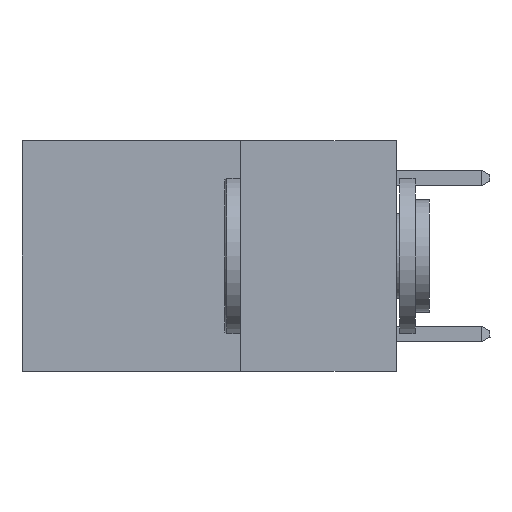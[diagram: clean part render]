
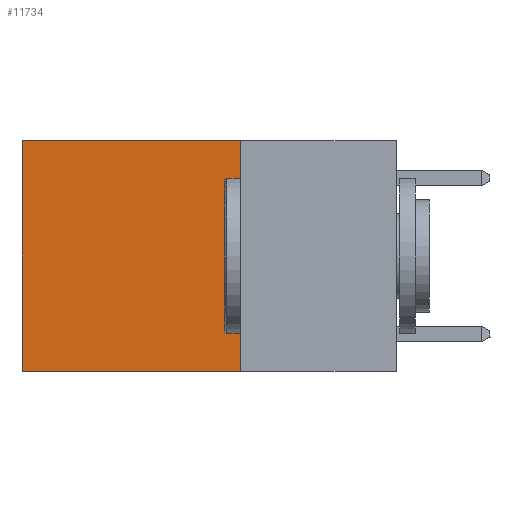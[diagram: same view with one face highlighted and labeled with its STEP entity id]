
A CAD part, left-side view. The second image highlights one B-rep face of the part: STEP entity #11734.
In plain terms, the highlighted planar face has unit normal (-1, 0, 0).
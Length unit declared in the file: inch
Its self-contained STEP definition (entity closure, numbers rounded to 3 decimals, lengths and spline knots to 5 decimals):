
#296 = CARTESIAN_POINT ( 'NONE',  ( 0.2625, 0.25, -0.37 ) ) ;
#345 = ORIENTED_EDGE ( 'NONE', *, *, #6903, .T. ) ;
#964 = DIRECTION ( 'NONE',  ( 0., 0., -1. ) ) ;
#1386 = CARTESIAN_POINT ( 'NONE',  ( 0.2625, 0.6, 0. ) ) ;
#1480 = LINE ( 'NONE', #13156, #5067 ) ;
#1482 = DIRECTION ( 'NONE',  ( 0., 0., -1. ) ) ;
#1592 = AXIS2_PLACEMENT_3D ( 'NONE', #18644, #15631, #6476 ) ;
#4390 = CARTESIAN_POINT ( 'NONE',  ( 0.2625, 0.25, 0. ) ) ;
#4649 = VERTEX_POINT ( 'NONE', #8957 ) ;
#4651 = VERTEX_POINT ( 'NONE', #4390 ) ;
#4912 = PLANE ( 'NONE',  #1592 ) ;
#5014 = CARTESIAN_POINT ( 'NONE',  ( 0.2625, 0.25, -0.37 ) ) ;
#5067 = VECTOR ( 'NONE', #964, 39.37008 ) ;
#5168 = EDGE_CURVE ( 'NONE', #13843, #4649, #1480, .T. ) ;
#6323 = VERTEX_POINT ( 'NONE', #5014 ) ;
#6476 = DIRECTION ( 'NONE',  ( 0., 0., -1. ) ) ;
#6615 = VECTOR ( 'NONE', #1482, 39.37008 ) ;
#6903 = EDGE_CURVE ( 'NONE', #4651, #13843, #7407, .T. ) ;
#6931 = VECTOR ( 'NONE', #9627, 39.37008 ) ;
#7346 = ORIENTED_EDGE ( 'NONE', *, *, #5168, .T. ) ;
#7407 = LINE ( 'NONE', #17249, #6931 ) ;
#7790 = FACE_OUTER_BOUND ( 'NONE', #17025, .T. ) ;
#8957 = CARTESIAN_POINT ( 'NONE',  ( 0.2625, 0.6, -0.37 ) ) ;
#9627 = DIRECTION ( 'NONE',  ( 0., 1., 0. ) ) ;
#10662 = CARTESIAN_POINT ( 'NONE',  ( 0.2625, 0.25, 0. ) ) ;
#10684 = LINE ( 'NONE', #10662, #6615 ) ;
#11107 = VECTOR ( 'NONE', #12575, 39.37008 ) ;
#11734 = ADVANCED_FACE ( 'NONE', ( #7790 ), #4912, .F. ) ;
#12575 = DIRECTION ( 'NONE',  ( 0., 1., 0. ) ) ;
#12589 = ORIENTED_EDGE ( 'NONE', *, *, #13375, .F. ) ;
#13156 = CARTESIAN_POINT ( 'NONE',  ( 0.2625, 0.6, 0. ) ) ;
#13375 = EDGE_CURVE ( 'NONE', #6323, #4649, #15638, .T. ) ;
#13843 = VERTEX_POINT ( 'NONE', #1386 ) ;
#15631 = DIRECTION ( 'NONE',  ( 1., 0., 0. ) ) ;
#15638 = LINE ( 'NONE', #296, #11107 ) ;
#17025 = EDGE_LOOP ( 'NONE', ( #7346, #12589, #17728, #345 ) ) ;
#17249 = CARTESIAN_POINT ( 'NONE',  ( 0.2625, 0.25, 0. ) ) ;
#17728 = ORIENTED_EDGE ( 'NONE', *, *, #18436, .F. ) ;
#18436 = EDGE_CURVE ( 'NONE', #4651, #6323, #10684, .T. ) ;
#18644 = CARTESIAN_POINT ( 'NONE',  ( 0.2625, 0.25, 0. ) ) ;
